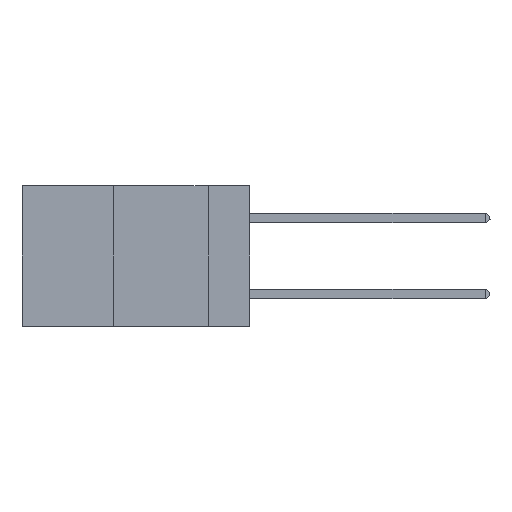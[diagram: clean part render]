
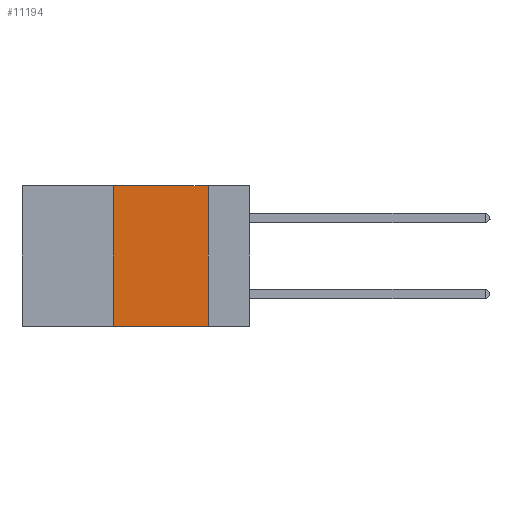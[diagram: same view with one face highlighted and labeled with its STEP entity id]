
A CAD part, left-side view. The second image highlights one B-rep face of the part: STEP entity #11194.
In plain terms, the highlighted planar face has unit normal (-1, 0, 0).
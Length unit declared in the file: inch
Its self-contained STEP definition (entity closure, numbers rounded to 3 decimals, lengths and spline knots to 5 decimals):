
#13 = FACE_OUTER_BOUND ( 'NONE', #6309, .T. ) ;
#495 = DIRECTION ( 'NONE',  ( 0., 0., -1. ) ) ;
#510 = EDGE_CURVE ( 'NONE', #671, #18360, #15810, .T. ) ;
#671 = VERTEX_POINT ( 'NONE', #1536 ) ;
#1062 = ORIENTED_EDGE ( 'NONE', *, *, #2550, .F. ) ;
#1097 = LINE ( 'NONE', #7543, #2903 ) ;
#1536 = CARTESIAN_POINT ( 'NONE',  ( 0., 0.36, -0.37 ) ) ;
#1671 = LINE ( 'NONE', #16580, #20892 ) ;
#1879 = LINE ( 'NONE', #21179, #17671 ) ;
#1974 = DIRECTION ( 'NONE',  ( 0., -1., 0. ) ) ;
#2550 = EDGE_CURVE ( 'NONE', #671, #3338, #1671, .T. ) ;
#2903 = VECTOR ( 'NONE', #495, 39.37008 ) ;
#3259 = AXIS2_PLACEMENT_3D ( 'NONE', #3454, #6459, #4758 ) ;
#3338 = VERTEX_POINT ( 'NONE', #11482 ) ;
#3454 = CARTESIAN_POINT ( 'NONE',  ( 0., 0.6, 0. ) ) ;
#4362 = ORIENTED_EDGE ( 'NONE', *, *, #7195, .F. ) ;
#4758 = DIRECTION ( 'NONE',  ( 0., 0., -1. ) ) ;
#6309 = EDGE_LOOP ( 'NONE', ( #4362, #10123, #1062, #9022 ) ) ;
#6459 = DIRECTION ( 'NONE',  ( 1., 0., 0. ) ) ;
#7195 = EDGE_CURVE ( 'NONE', #13466, #18360, #1097, .T. ) ;
#7543 = CARTESIAN_POINT ( 'NONE',  ( 0., 0.11, 0. ) ) ;
#7583 = VECTOR ( 'NONE', #20526, 39.37008 ) ;
#9022 = ORIENTED_EDGE ( 'NONE', *, *, #510, .T. ) ;
#9814 = PLANE ( 'NONE',  #3259 ) ;
#10123 = ORIENTED_EDGE ( 'NONE', *, *, #12073, .F. ) ;
#11194 = ADVANCED_FACE ( 'NONE', ( #13 ), #9814, .F. ) ;
#11349 = DIRECTION ( 'NONE',  ( 0., 0., 1. ) ) ;
#11482 = CARTESIAN_POINT ( 'NONE',  ( 0., 0.36, 0. ) ) ;
#11899 = CARTESIAN_POINT ( 'NONE',  ( 0., 0.11, 0. ) ) ;
#12073 = EDGE_CURVE ( 'NONE', #3338, #13466, #1879, .T. ) ;
#13466 = VERTEX_POINT ( 'NONE', #11899 ) ;
#15810 = LINE ( 'NONE', #20847, #7583 ) ;
#16580 = CARTESIAN_POINT ( 'NONE',  ( 0., 0.36, 0. ) ) ;
#17671 = VECTOR ( 'NONE', #1974, 39.37008 ) ;
#18360 = VERTEX_POINT ( 'NONE', #20707 ) ;
#20526 = DIRECTION ( 'NONE',  ( 0., -1., 0. ) ) ;
#20707 = CARTESIAN_POINT ( 'NONE',  ( 0., 0.11, -0.37 ) ) ;
#20847 = CARTESIAN_POINT ( 'NONE',  ( 0., 0.6, -0.37 ) ) ;
#20892 = VECTOR ( 'NONE', #11349, 39.37008 ) ;
#21179 = CARTESIAN_POINT ( 'NONE',  ( 0., 0.6, 0. ) ) ;
